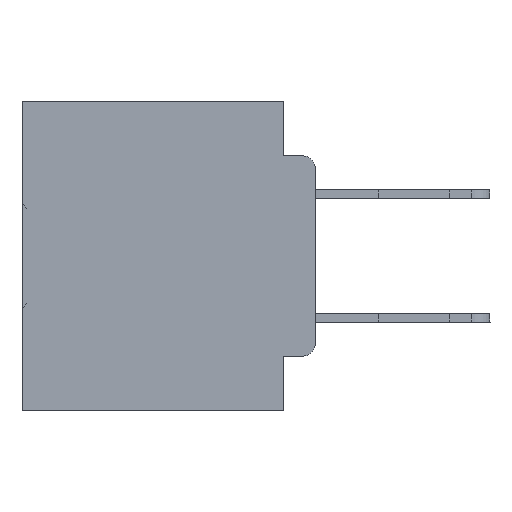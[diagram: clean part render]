
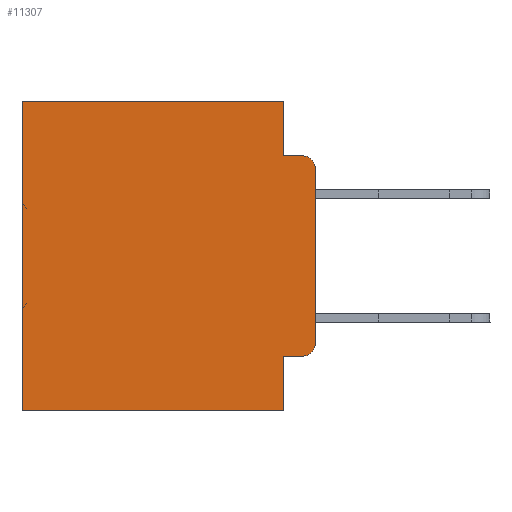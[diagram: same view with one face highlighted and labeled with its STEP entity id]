
A CAD part, left-side view. The second image highlights one B-rep face of the part: STEP entity #11307.
In plain terms, the highlighted planar face has unit normal (-1, 0, 0).
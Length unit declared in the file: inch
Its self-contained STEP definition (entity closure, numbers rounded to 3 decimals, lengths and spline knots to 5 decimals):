
#2289 = CARTESIAN_POINT ( 'NONE',  ( 0.298, 0.02, -0.3915 ) ) ;
#2405 = DIRECTION ( 'NONE',  ( 0., 0., -1. ) ) ;
#2440 = CARTESIAN_POINT ( 'NONE',  ( 0.298, 0.051, -0.0885 ) ) ;
#3155 = EDGE_LOOP ( 'NONE', ( #15019, #30912, #25163, #30693, #13860, #34292, #23897, #19596, #7648, #24235 ) ) ;
#3852 = LINE ( 'NONE', #8102, #22698 ) ;
#4380 = PLANE ( 'NONE',  #25584 ) ;
#4630 = CIRCLE ( 'NONE', #16839, 0.02 ) ;
#5609 = VERTEX_POINT ( 'NONE', #2440 ) ;
#6095 = LINE ( 'NONE', #25161, #14904 ) ;
#6348 = EDGE_CURVE ( 'NONE', #14852, #5609, #18606, .T. ) ;
#7616 = DIRECTION ( 'NONE',  ( -1., 0., 0. ) ) ;
#7648 = ORIENTED_EDGE ( 'NONE', *, *, #8975, .T. ) ;
#7813 = VERTEX_POINT ( 'NONE', #12024 ) ;
#8102 = CARTESIAN_POINT ( 'NONE',  ( 0.298, 0., -0.5 ) ) ;
#8207 = EDGE_CURVE ( 'NONE', #28730, #9764, #6095, .T. ) ;
#8975 = EDGE_CURVE ( 'NONE', #35139, #35878, #29779, .T. ) ;
#9118 = DIRECTION ( 'NONE',  ( 0., -1., 0. ) ) ;
#9764 = VERTEX_POINT ( 'NONE', #16302 ) ;
#10030 = VECTOR ( 'NONE', #9118, 39.37008 ) ;
#11272 = CARTESIAN_POINT ( 'NONE',  ( 0.298, 0.473, -0.5 ) ) ;
#11307 = ADVANCED_FACE ( 'NONE', ( #36187 ), #4380, .F. ) ;
#11599 = DIRECTION ( 'NONE',  ( 0., 0., -1. ) ) ;
#12024 = CARTESIAN_POINT ( 'NONE',  ( 0.298, 0.051, -0.5 ) ) ;
#12310 = CARTESIAN_POINT ( 'NONE',  ( 0.298, 0.02, -0.0885 ) ) ;
#12436 = CARTESIAN_POINT ( 'NONE',  ( 0.298, 0.051, -0.4115 ) ) ;
#12839 = DIRECTION ( 'NONE',  ( 0., 1., 0. ) ) ;
#13860 = ORIENTED_EDGE ( 'NONE', *, *, #20057, .T. ) ;
#14005 = CARTESIAN_POINT ( 'NONE',  ( 0.298, 0.051, -0.4115 ) ) ;
#14321 = DIRECTION ( 'NONE',  ( 1., 0., 0. ) ) ;
#14734 = CARTESIAN_POINT ( 'NONE',  ( 0.298, 0.051, 0. ) ) ;
#14852 = VERTEX_POINT ( 'NONE', #28111 ) ;
#14904 = VECTOR ( 'NONE', #33632, 39.37008 ) ;
#15019 = ORIENTED_EDGE ( 'NONE', *, *, #8207, .F. ) ;
#15276 = EDGE_CURVE ( 'NONE', #21381, #33208, #32525, .T. ) ;
#15325 = CIRCLE ( 'NONE', #19690, 0.02 ) ;
#16302 = CARTESIAN_POINT ( 'NONE',  ( 0.298, 0., -0.3915 ) ) ;
#16344 = DIRECTION ( 'NONE',  ( -1., 0., 0. ) ) ;
#16767 = EDGE_CURVE ( 'NONE', #35139, #7813, #25791, .T. ) ;
#16839 = AXIS2_PLACEMENT_3D ( 'NONE', #35963, #7616, #30073 ) ;
#18187 = CARTESIAN_POINT ( 'NONE',  ( 0.298, 0.473, 0. ) ) ;
#18446 = EDGE_CURVE ( 'NONE', #28730, #22694, #4630, .T. ) ;
#18606 = LINE ( 'NONE', #14734, #31749 ) ;
#19362 = VECTOR ( 'NONE', #11599, 39.37008 ) ;
#19429 = CARTESIAN_POINT ( 'NONE',  ( 0.298, 0.051, 0. ) ) ;
#19596 = ORIENTED_EDGE ( 'NONE', *, *, #16767, .F. ) ;
#19690 = AXIS2_PLACEMENT_3D ( 'NONE', #2289, #16344, #2405 ) ;
#20057 = EDGE_CURVE ( 'NONE', #14852, #21381, #34528, .T. ) ;
#21381 = VERTEX_POINT ( 'NONE', #26251 ) ;
#21441 = VECTOR ( 'NONE', #33532, 39.37008 ) ;
#22689 = VECTOR ( 'NONE', #12839, 39.37008 ) ;
#22694 = VERTEX_POINT ( 'NONE', #12310 ) ;
#22698 = VECTOR ( 'NONE', #24608, 39.37008 ) ;
#23897 = ORIENTED_EDGE ( 'NONE', *, *, #31041, .F. ) ;
#24182 = CARTESIAN_POINT ( 'NONE',  ( 0.298, 0.051, -0.0885 ) ) ;
#24235 = ORIENTED_EDGE ( 'NONE', *, *, #28525, .T. ) ;
#24608 = DIRECTION ( 'NONE',  ( 0., 1., 0. ) ) ;
#25161 = CARTESIAN_POINT ( 'NONE',  ( 0.298, 0., 0. ) ) ;
#25163 = ORIENTED_EDGE ( 'NONE', *, *, #29658, .F. ) ;
#25434 = VECTOR ( 'NONE', #29433, 39.37008 ) ;
#25584 = AXIS2_PLACEMENT_3D ( 'NONE', #32533, #14321, #30885 ) ;
#25791 = LINE ( 'NONE', #19429, #21441 ) ;
#26136 = DIRECTION ( 'NONE',  ( 0., 0., -1. ) ) ;
#26251 = CARTESIAN_POINT ( 'NONE',  ( 0.298, 0.473, 0. ) ) ;
#28111 = CARTESIAN_POINT ( 'NONE',  ( 0.298, 0.051, 0. ) ) ;
#28142 = CARTESIAN_POINT ( 'NONE',  ( 0.298, 0., -0.1085 ) ) ;
#28525 = EDGE_CURVE ( 'NONE', #35878, #9764, #15325, .T. ) ;
#28730 = VERTEX_POINT ( 'NONE', #28142 ) ;
#29133 = CARTESIAN_POINT ( 'NONE',  ( 0.298, 0.02, -0.4115 ) ) ;
#29433 = DIRECTION ( 'NONE',  ( 0., -1., 0. ) ) ;
#29640 = CARTESIAN_POINT ( 'NONE',  ( 0.298, 0., 0. ) ) ;
#29658 = EDGE_CURVE ( 'NONE', #5609, #22694, #31124, .T. ) ;
#29779 = LINE ( 'NONE', #12436, #10030 ) ;
#30073 = DIRECTION ( 'NONE',  ( 0., 0., -1. ) ) ;
#30693 = ORIENTED_EDGE ( 'NONE', *, *, #6348, .F. ) ;
#30885 = DIRECTION ( 'NONE',  ( 0., 0., -1. ) ) ;
#30912 = ORIENTED_EDGE ( 'NONE', *, *, #18446, .T. ) ;
#31041 = EDGE_CURVE ( 'NONE', #7813, #33208, #3852, .T. ) ;
#31124 = LINE ( 'NONE', #24182, #25434 ) ;
#31749 = VECTOR ( 'NONE', #26136, 39.37008 ) ;
#32525 = LINE ( 'NONE', #18187, #19362 ) ;
#32533 = CARTESIAN_POINT ( 'NONE',  ( 0.298, 0., 0. ) ) ;
#33208 = VERTEX_POINT ( 'NONE', #11272 ) ;
#33532 = DIRECTION ( 'NONE',  ( 0., 0., -1. ) ) ;
#33632 = DIRECTION ( 'NONE',  ( 0., 0., -1. ) ) ;
#34292 = ORIENTED_EDGE ( 'NONE', *, *, #15276, .T. ) ;
#34528 = LINE ( 'NONE', #29640, #22689 ) ;
#35139 = VERTEX_POINT ( 'NONE', #14005 ) ;
#35878 = VERTEX_POINT ( 'NONE', #29133 ) ;
#35963 = CARTESIAN_POINT ( 'NONE',  ( 0.298, 0.02, -0.1085 ) ) ;
#36187 = FACE_OUTER_BOUND ( 'NONE', #3155, .T. ) ;
